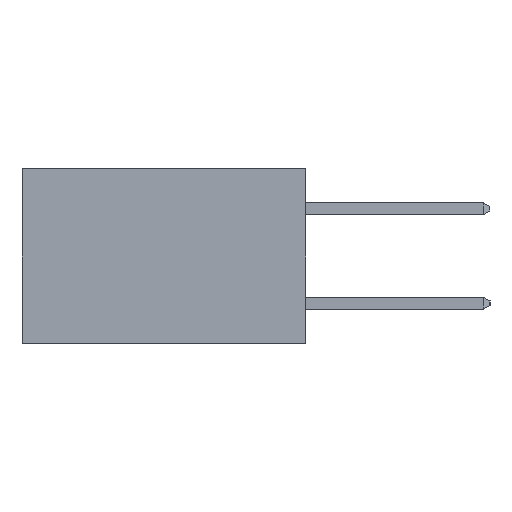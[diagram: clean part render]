
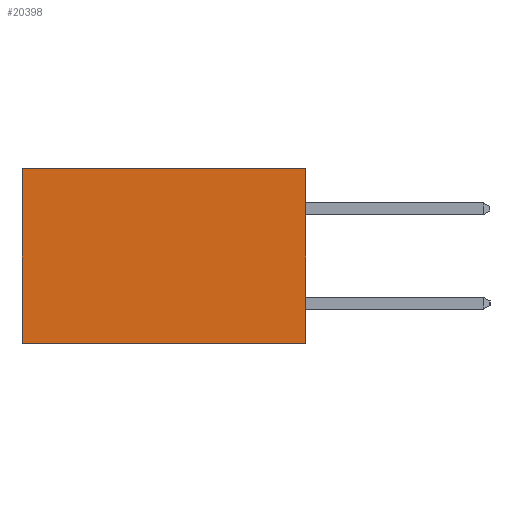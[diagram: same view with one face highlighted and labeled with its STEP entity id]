
A CAD part, left-side view. The second image highlights one B-rep face of the part: STEP entity #20398.
In plain terms, the highlighted planar face has unit normal (-1, 0, 0).
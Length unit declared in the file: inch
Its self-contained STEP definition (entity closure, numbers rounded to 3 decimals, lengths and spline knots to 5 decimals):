
#1222 = CARTESIAN_POINT ( 'NONE',  ( 0.2615, 0., 0. ) ) ;
#1627 = EDGE_CURVE ( 'NONE', #14236, #2020, #1675, .T. ) ;
#1675 = LINE ( 'NONE', #18775, #21000 ) ;
#2020 = VERTEX_POINT ( 'NONE', #8512 ) ;
#2960 = VERTEX_POINT ( 'NONE', #17080 ) ;
#3015 = EDGE_CURVE ( 'NONE', #2960, #10944, #6466, .T. ) ;
#3035 = EDGE_LOOP ( 'NONE', ( #9278, #4406, #5927, #7282 ) ) ;
#3750 = FACE_OUTER_BOUND ( 'NONE', #3035, .T. ) ;
#4406 = ORIENTED_EDGE ( 'NONE', *, *, #12774, .F. ) ;
#5293 = VECTOR ( 'NONE', #12847, 39.37008 ) ;
#5927 = ORIENTED_EDGE ( 'NONE', *, *, #3015, .F. ) ;
#6466 = LINE ( 'NONE', #13686, #5293 ) ;
#6628 = VECTOR ( 'NONE', #8714, 39.37008 ) ;
#7114 = VECTOR ( 'NONE', #11189, 39.37008 ) ;
#7219 = LINE ( 'NONE', #1222, #6628 ) ;
#7282 = ORIENTED_EDGE ( 'NONE', *, *, #21836, .T. ) ;
#8512 = CARTESIAN_POINT ( 'NONE',  ( 0.2615, 0.6, -0.37 ) ) ;
#8714 = DIRECTION ( 'NONE',  ( 0., 1., 0. ) ) ;
#8916 = LINE ( 'NONE', #24132, #7114 ) ;
#9278 = ORIENTED_EDGE ( 'NONE', *, *, #1627, .T. ) ;
#10748 = CARTESIAN_POINT ( 'NONE',  ( 0.2615, 0., -0.37 ) ) ;
#10944 = VERTEX_POINT ( 'NONE', #23812 ) ;
#11189 = DIRECTION ( 'NONE',  ( 0., 1., 0. ) ) ;
#12637 = DIRECTION ( 'NONE',  ( 0., 0., -1. ) ) ;
#12774 = EDGE_CURVE ( 'NONE', #10944, #2020, #8916, .T. ) ;
#12847 = DIRECTION ( 'NONE',  ( 0., 0., -1. ) ) ;
#13686 = CARTESIAN_POINT ( 'NONE',  ( 0.2615, 0., -0.37 ) ) ;
#14236 = VERTEX_POINT ( 'NONE', #17834 ) ;
#17080 = CARTESIAN_POINT ( 'NONE',  ( 0.2615, 0., 0. ) ) ;
#17834 = CARTESIAN_POINT ( 'NONE',  ( 0.2615, 0.6, 0. ) ) ;
#18539 = DIRECTION ( 'NONE',  ( 0., 0., -1. ) ) ;
#18775 = CARTESIAN_POINT ( 'NONE',  ( 0.2615, 0.6, -0.37 ) ) ;
#19975 = PLANE ( 'NONE',  #22785 ) ;
#20398 = ADVANCED_FACE ( 'NONE', ( #3750 ), #19975, .F. ) ;
#21000 = VECTOR ( 'NONE', #18539, 39.37008 ) ;
#21836 = EDGE_CURVE ( 'NONE', #2960, #14236, #7219, .T. ) ;
#22785 = AXIS2_PLACEMENT_3D ( 'NONE', #10748, #23697, #12637 ) ;
#23697 = DIRECTION ( 'NONE',  ( 1., 0., 0. ) ) ;
#23812 = CARTESIAN_POINT ( 'NONE',  ( 0.2615, 0., -0.37 ) ) ;
#24132 = CARTESIAN_POINT ( 'NONE',  ( 0.2615, 0., -0.37 ) ) ;
